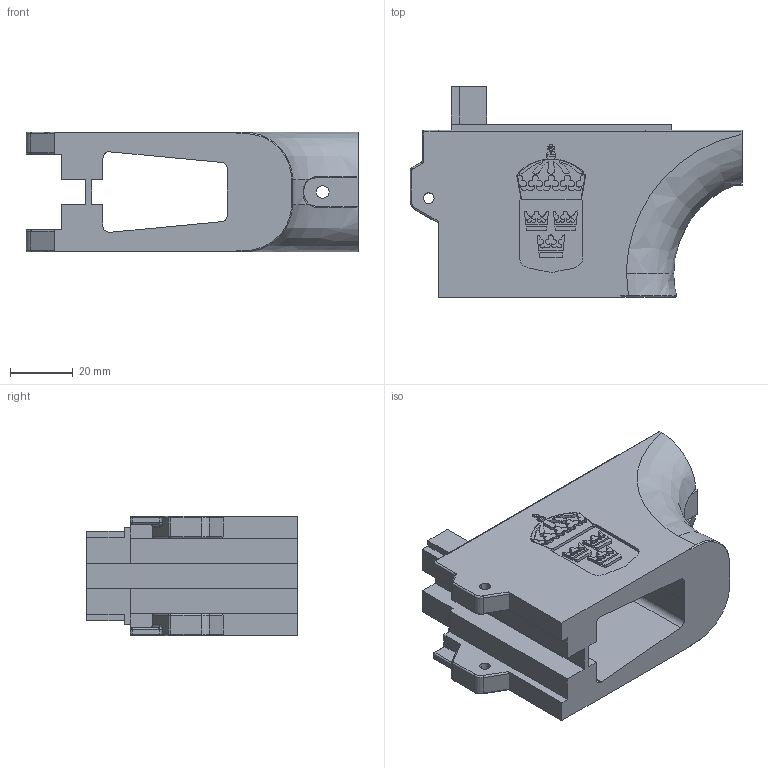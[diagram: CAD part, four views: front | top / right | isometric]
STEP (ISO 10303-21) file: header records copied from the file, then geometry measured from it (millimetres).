
FILE_DESCRIPTION (( 'STEP AP214' ), '1' );
FILE_NAME ('magwell_m45_sweden.STEP', '2020-10-09T21:10:15', ( '' ), ( '' ), 'SwSTEP 2.0', 'SolidWorks 2020', '' );
FILE_SCHEMA (( 'AUTOMOTIVE_DESIGN' ));
Length unit declared in the file: millimetre
Products named in the file (1): magwell_m45_sweden
Bounding box: 105.51 x 66.9 x 38 mm (x, y, z)
Volume: 113687.3 mm3; surface area: 29156.8 mm2
Topology: 1 solids, 2 shells, 488 faces, 1363 edges, 886 vertices
Faces by surface type: bspline 246, plane 190, cylinder 50, cone 2
Entity records: 18211 total; most frequent: CARTESIAN_POINT 7578, ORIENTED_EDGE 2706, EDGE_CURVE 1353, DIRECTION 1335, VERTEX_POINT 886, LINE 661, VECTOR 661, B_SPLINE_CURVE_WITH_KNOTS 578
